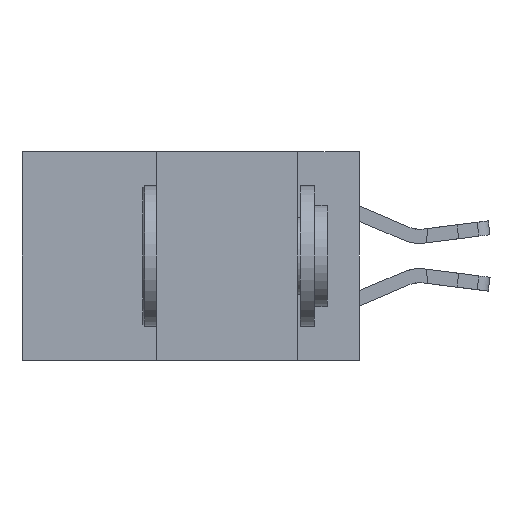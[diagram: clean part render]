
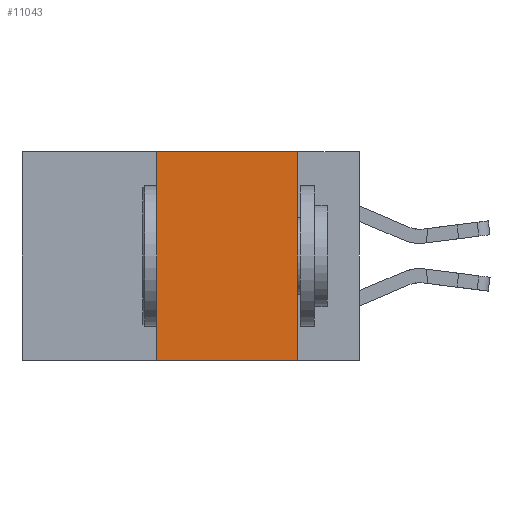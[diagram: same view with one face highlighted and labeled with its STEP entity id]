
A CAD part, left-side view. The second image highlights one B-rep face of the part: STEP entity #11043.
In plain terms, the highlighted planar face has unit normal (-1, 0, 0).
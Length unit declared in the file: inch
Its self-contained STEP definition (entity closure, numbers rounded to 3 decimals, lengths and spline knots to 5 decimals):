
#66 = VECTOR ( 'NONE', #8632, 39.37008 ) ;
#216 = VERTEX_POINT ( 'NONE', #7372 ) ;
#1150 = DIRECTION ( 'NONE',  ( 0., -1., 0. ) ) ;
#1434 = CARTESIAN_POINT ( 'NONE',  ( 0., 0.6, 0. ) ) ;
#2860 = LINE ( 'NONE', #1434, #10508 ) ;
#3756 = LINE ( 'NONE', #12177, #11854 ) ;
#5333 = EDGE_CURVE ( 'NONE', #15443, #216, #2860, .T. ) ;
#5608 = CARTESIAN_POINT ( 'NONE',  ( 0., 0.36, 0. ) ) ;
#6158 = EDGE_CURVE ( 'NONE', #6893, #18768, #3756, .T. ) ;
#6893 = VERTEX_POINT ( 'NONE', #16821 ) ;
#7083 = CARTESIAN_POINT ( 'NONE',  ( 0., 0.36, 0. ) ) ;
#7235 = ORIENTED_EDGE ( 'NONE', *, *, #5333, .F. ) ;
#7372 = CARTESIAN_POINT ( 'NONE',  ( 0., 0.11, 0. ) ) ;
#7621 = VECTOR ( 'NONE', #15693, 39.37008 ) ;
#8182 = LINE ( 'NONE', #7083, #66 ) ;
#8301 = CARTESIAN_POINT ( 'NONE',  ( 0., 0.6, 0. ) ) ;
#8366 = PLANE ( 'NONE',  #11089 ) ;
#8632 = DIRECTION ( 'NONE',  ( 0., 0., 1. ) ) ;
#9138 = CARTESIAN_POINT ( 'NONE',  ( 0., 0.11, -0.37 ) ) ;
#9633 = CARTESIAN_POINT ( 'NONE',  ( 0., 0.11, 0. ) ) ;
#9661 = FACE_OUTER_BOUND ( 'NONE', #14958, .T. ) ;
#9878 = DIRECTION ( 'NONE',  ( 0., 0., -1. ) ) ;
#10508 = VECTOR ( 'NONE', #1150, 39.37008 ) ;
#11043 = ADVANCED_FACE ( 'NONE', ( #9661 ), #8366, .F. ) ;
#11089 = AXIS2_PLACEMENT_3D ( 'NONE', #8301, #19025, #9878 ) ;
#11854 = VECTOR ( 'NONE', #13723, 39.37008 ) ;
#12177 = CARTESIAN_POINT ( 'NONE',  ( 0., 0.6, -0.37 ) ) ;
#13161 = EDGE_CURVE ( 'NONE', #6893, #15443, #8182, .T. ) ;
#13723 = DIRECTION ( 'NONE',  ( 0., -1., 0. ) ) ;
#14843 = EDGE_CURVE ( 'NONE', #216, #18768, #15668, .T. ) ;
#14958 = EDGE_LOOP ( 'NONE', ( #18914, #7235, #15286, #19415 ) ) ;
#15286 = ORIENTED_EDGE ( 'NONE', *, *, #13161, .F. ) ;
#15443 = VERTEX_POINT ( 'NONE', #5608 ) ;
#15668 = LINE ( 'NONE', #9633, #7621 ) ;
#15693 = DIRECTION ( 'NONE',  ( 0., 0., -1. ) ) ;
#16821 = CARTESIAN_POINT ( 'NONE',  ( 0., 0.36, -0.37 ) ) ;
#18768 = VERTEX_POINT ( 'NONE', #9138 ) ;
#18914 = ORIENTED_EDGE ( 'NONE', *, *, #14843, .F. ) ;
#19025 = DIRECTION ( 'NONE',  ( 1., 0., 0. ) ) ;
#19415 = ORIENTED_EDGE ( 'NONE', *, *, #6158, .T. ) ;
